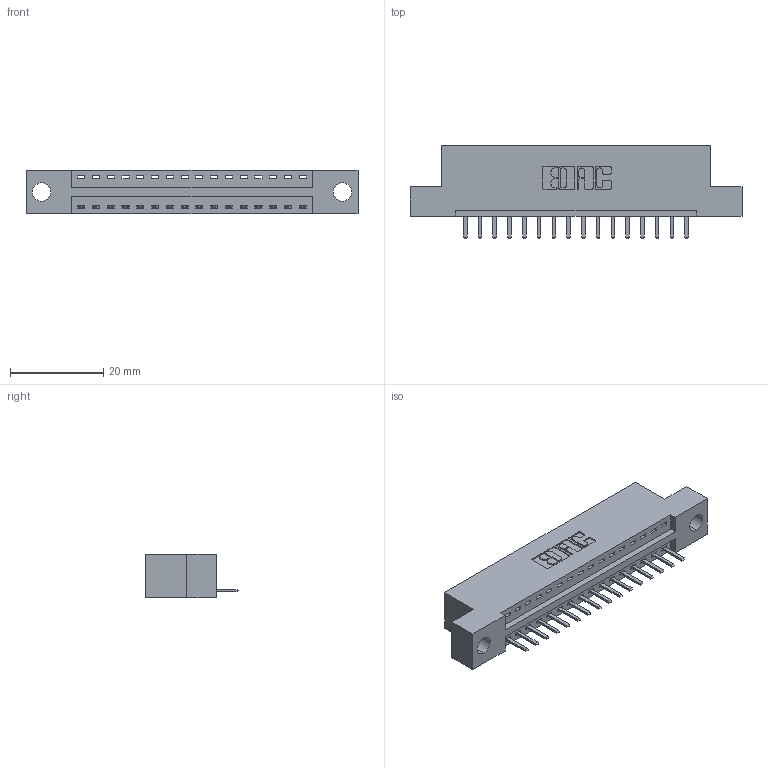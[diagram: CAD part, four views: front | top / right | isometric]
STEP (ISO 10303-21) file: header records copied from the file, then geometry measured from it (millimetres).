
FILE_DESCRIPTION (( 'STEP AP203' ), '1' );
FILE_NAME ('396-016-520-104.STEP', '2018-08-31T22:22:54', ( '' ), ( '' ), 'SwSTEP 2.0', 'SolidWorks 2016', '' );
FILE_SCHEMA (( 'CONFIG_CONTROL_DESIGN' ));
Length unit declared in the file: inch
Products named in the file (3): 346 Part_Flush Mounting Lugs - 0.156 Dia-TH; 345-292-001_345-293-120; 396-016-520-104
Assembly tree (17 placements, depth 2):
  396-016-520-104
    346 Part_Flush Mounting Lugs - 0.156 Dia-TH
    345-292-001_345-293-120  x16
Bounding box: 71.37 x 20.02 x 9.4 mm (x, y, z)
Volume: 6519.1 mm3; surface area: 7518.7 mm2
Topology: 17 solids, 17 shells, 1114 faces, 3273 edges, 2138 vertices
Faces by surface type: plane 748, cylinder 366
Entity records: 13547 total; most frequent: CARTESIAN_POINT 2348, ORIENTED_EDGE 2286, DIRECTION 2091, EDGE_CURVE 1143, LINE 943, VECTOR 943, VERTEX_POINT 758, AXIS2_PLACEMENT_3D 574
